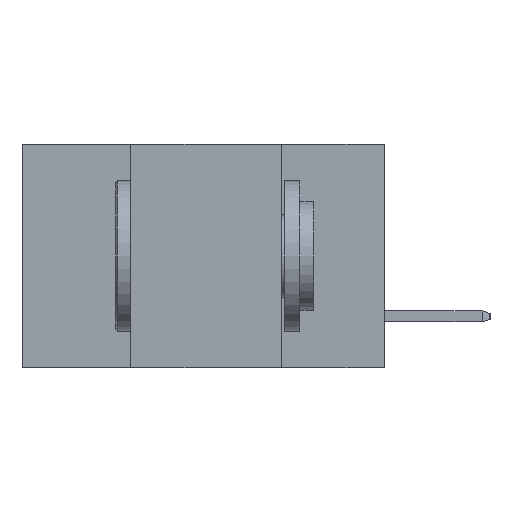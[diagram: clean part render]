
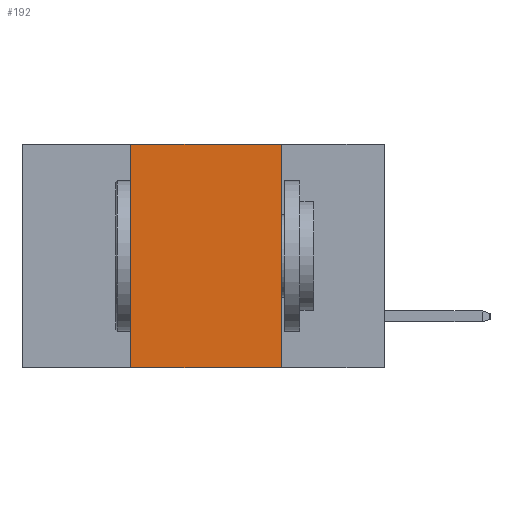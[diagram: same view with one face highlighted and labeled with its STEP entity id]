
A CAD part, left-side view. The second image highlights one B-rep face of the part: STEP entity #192.
In plain terms, the highlighted planar face has unit normal (-1, 0, 0).
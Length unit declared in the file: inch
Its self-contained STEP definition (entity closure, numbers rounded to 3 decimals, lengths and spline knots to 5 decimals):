
#75 = DIRECTION ( 'NONE',  ( 0., -1., 0. ) ) ;
#118 = CARTESIAN_POINT ( 'NONE',  ( 0., 0.6, -0.37 ) ) ;
#192 = ADVANCED_FACE ( 'NONE', ( #13167 ), #6162, .F. ) ;
#297 = VECTOR ( 'NONE', #13849, 39.37008 ) ;
#918 = LINE ( 'NONE', #16471, #4051 ) ;
#931 = DIRECTION ( 'NONE',  ( 0., 0., 1. ) ) ;
#940 = CARTESIAN_POINT ( 'NONE',  ( 0., 0.17, 0. ) ) ;
#1688 = VERTEX_POINT ( 'NONE', #940 ) ;
#2051 = LINE ( 'NONE', #118, #8625 ) ;
#2524 = CARTESIAN_POINT ( 'NONE',  ( 0., 0.42, 0. ) ) ;
#2550 = CARTESIAN_POINT ( 'NONE',  ( 0., 0.6, 0. ) ) ;
#2672 = CARTESIAN_POINT ( 'NONE',  ( 0., 0.42, -0.37 ) ) ;
#3315 = VERTEX_POINT ( 'NONE', #3739 ) ;
#3485 = CARTESIAN_POINT ( 'NONE',  ( 0., 0.6, 0. ) ) ;
#3739 = CARTESIAN_POINT ( 'NONE',  ( 0., 0.17, -0.37 ) ) ;
#3866 = VERTEX_POINT ( 'NONE', #2672 ) ;
#4051 = VECTOR ( 'NONE', #931, 39.37008 ) ;
#5244 = ORIENTED_EDGE ( 'NONE', *, *, #8966, .T. ) ;
#6162 = PLANE ( 'NONE',  #15431 ) ;
#6373 = DIRECTION ( 'NONE',  ( 0., 0., -1. ) ) ;
#6906 = LINE ( 'NONE', #10250, #9948 ) ;
#7328 = LINE ( 'NONE', #3485, #297 ) ;
#8625 = VECTOR ( 'NONE', #75, 39.37008 ) ;
#8653 = ORIENTED_EDGE ( 'NONE', *, *, #11832, .F. ) ;
#8966 = EDGE_CURVE ( 'NONE', #3866, #3315, #2051, .T. ) ;
#9831 = EDGE_LOOP ( 'NONE', ( #11637, #8653, #16465, #5244 ) ) ;
#9948 = VECTOR ( 'NONE', #6373, 39.37008 ) ;
#10250 = CARTESIAN_POINT ( 'NONE',  ( 0., 0.17, 0. ) ) ;
#11214 = EDGE_CURVE ( 'NONE', #3866, #14351, #918, .T. ) ;
#11525 = DIRECTION ( 'NONE',  ( 1., 0., 0. ) ) ;
#11637 = ORIENTED_EDGE ( 'NONE', *, *, #12486, .F. ) ;
#11832 = EDGE_CURVE ( 'NONE', #14351, #1688, #7328, .T. ) ;
#12486 = EDGE_CURVE ( 'NONE', #1688, #3315, #6906, .T. ) ;
#12966 = DIRECTION ( 'NONE',  ( 0., 0., -1. ) ) ;
#13167 = FACE_OUTER_BOUND ( 'NONE', #9831, .T. ) ;
#13849 = DIRECTION ( 'NONE',  ( 0., -1., 0. ) ) ;
#14351 = VERTEX_POINT ( 'NONE', #2524 ) ;
#15431 = AXIS2_PLACEMENT_3D ( 'NONE', #2550, #11525, #12966 ) ;
#16465 = ORIENTED_EDGE ( 'NONE', *, *, #11214, .F. ) ;
#16471 = CARTESIAN_POINT ( 'NONE',  ( 0., 0.42, 0. ) ) ;
